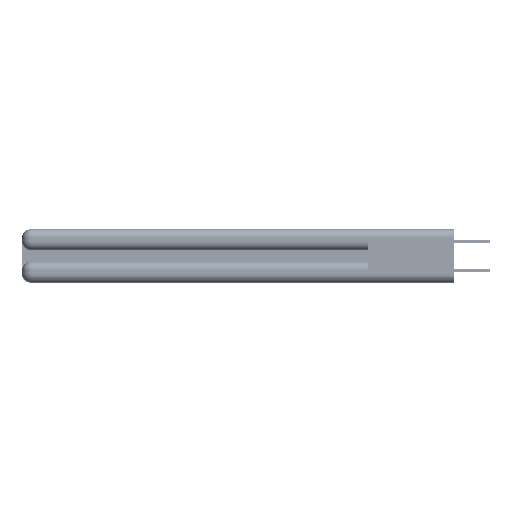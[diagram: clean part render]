
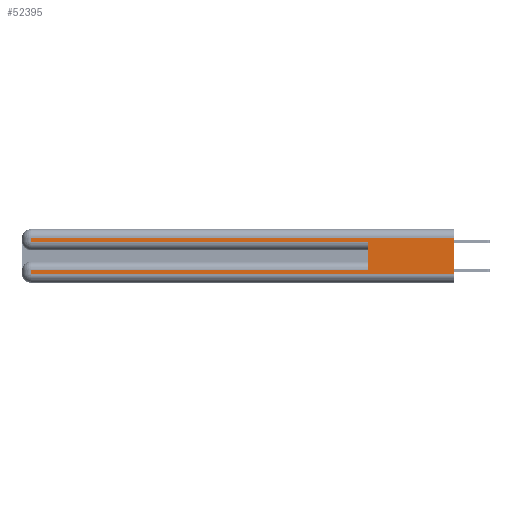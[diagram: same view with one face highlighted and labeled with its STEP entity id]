
A CAD part, left-side view. The second image highlights one B-rep face of the part: STEP entity #52395.
In plain terms, the highlighted planar face has unit normal (-1, 0, 0).
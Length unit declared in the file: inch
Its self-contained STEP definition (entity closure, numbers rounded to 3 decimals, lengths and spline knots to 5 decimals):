
#705 = CARTESIAN_POINT ( 'NONE',  ( 0., 0., 0.085 ) ) ;
#1115 = CARTESIAN_POINT ( 'NONE',  ( 0., 2.94, 0.37 ) ) ;
#1742 = DIRECTION ( 'NONE',  ( 0., 1., 0. ) ) ;
#2378 = VECTOR ( 'NONE', #22180, 39.37008 ) ;
#3705 = ORIENTED_EDGE ( 'NONE', *, *, #5007, .F. ) ;
#4146 = VERTEX_POINT ( 'NONE', #29857 ) ;
#4688 = DIRECTION ( 'NONE',  ( 1., 0., 0. ) ) ;
#5005 = VERTEX_POINT ( 'NONE', #43835 ) ;
#5007 = EDGE_CURVE ( 'NONE', #45916, #56265, #9834, .T. ) ;
#7320 = EDGE_CURVE ( 'NONE', #31704, #20163, #23789, .T. ) ;
#8880 = CARTESIAN_POINT ( 'NONE',  ( 0., 0.6, 0.145 ) ) ;
#9250 = PLANE ( 'NONE',  #31432 ) ;
#9301 = VECTOR ( 'NONE', #55175, 39.37008 ) ;
#9562 = CARTESIAN_POINT ( 'NONE',  ( 0., 2.94, 0.085 ) ) ;
#9834 = LINE ( 'NONE', #8880, #2378 ) ;
#10507 = ORIENTED_EDGE ( 'NONE', *, *, #16916, .T. ) ;
#10761 = CARTESIAN_POINT ( 'NONE',  ( 0., 0., 0.285 ) ) ;
#11599 = ORIENTED_EDGE ( 'NONE', *, *, #7320, .T. ) ;
#13138 = ORIENTED_EDGE ( 'NONE', *, *, #31001, .T. ) ;
#13433 = DIRECTION ( 'NONE',  ( 0., 0., -1. ) ) ;
#13495 = ORIENTED_EDGE ( 'NONE', *, *, #27789, .F. ) ;
#13810 = DIRECTION ( 'NONE',  ( 0., 1., 0. ) ) ;
#15706 = VECTOR ( 'NONE', #40473, 39.37008 ) ;
#16916 = EDGE_CURVE ( 'NONE', #33197, #56265, #39245, .T. ) ;
#17334 = CARTESIAN_POINT ( 'NONE',  ( 0., 0., 0.06 ) ) ;
#18394 = DIRECTION ( 'NONE',  ( 0., 0., -1. ) ) ;
#18413 = LINE ( 'NONE', #1115, #15706 ) ;
#18759 = CARTESIAN_POINT ( 'NONE',  ( 0., 0., 0.37 ) ) ;
#20163 = VERTEX_POINT ( 'NONE', #44011 ) ;
#22098 = LINE ( 'NONE', #27802, #38376 ) ;
#22180 = DIRECTION ( 'NONE',  ( 0., 0., 1. ) ) ;
#23002 = LINE ( 'NONE', #18759, #35207 ) ;
#23789 = LINE ( 'NONE', #43798, #40085 ) ;
#26553 = CARTESIAN_POINT ( 'NONE',  ( 0., 0., 0.37 ) ) ;
#27789 = EDGE_CURVE ( 'NONE', #55184, #4146, #23002, .T. ) ;
#27802 = CARTESIAN_POINT ( 'NONE',  ( 0., 0., 0.31 ) ) ;
#27840 = EDGE_LOOP ( 'NONE', ( #13495, #29357, #37471, #10507, #3705, #13138, #11599, #28764 ) ) ;
#28746 = EDGE_CURVE ( 'NONE', #20163, #4146, #48695, .T. ) ;
#28764 = ORIENTED_EDGE ( 'NONE', *, *, #28746, .T. ) ;
#29357 = ORIENTED_EDGE ( 'NONE', *, *, #53196, .T. ) ;
#29857 = CARTESIAN_POINT ( 'NONE',  ( 0., 0., 0.06 ) ) ;
#30088 = CARTESIAN_POINT ( 'NONE',  ( 0., 0., 0.31 ) ) ;
#30915 = FACE_OUTER_BOUND ( 'NONE', #27840, .T. ) ;
#31001 = EDGE_CURVE ( 'NONE', #45916, #31704, #46957, .T. ) ;
#31432 = AXIS2_PLACEMENT_3D ( 'NONE', #26553, #4688, #13433 ) ;
#31704 = VERTEX_POINT ( 'NONE', #9562 ) ;
#32636 = CARTESIAN_POINT ( 'NONE',  ( 0., 0.6, 0.285 ) ) ;
#33059 = VECTOR ( 'NONE', #38817, 39.37008 ) ;
#33197 = VERTEX_POINT ( 'NONE', #41361 ) ;
#35207 = VECTOR ( 'NONE', #18394, 39.37008 ) ;
#37471 = ORIENTED_EDGE ( 'NONE', *, *, #48840, .T. ) ;
#38376 = VECTOR ( 'NONE', #1742, 39.37008 ) ;
#38817 = DIRECTION ( 'NONE',  ( 0., -1., 0. ) ) ;
#39245 = LINE ( 'NONE', #10761, #9301 ) ;
#40085 = VECTOR ( 'NONE', #52514, 39.37008 ) ;
#40473 = DIRECTION ( 'NONE',  ( 0., 0., -1. ) ) ;
#41361 = CARTESIAN_POINT ( 'NONE',  ( 0., 2.94, 0.285 ) ) ;
#43798 = CARTESIAN_POINT ( 'NONE',  ( 0., 2.94, 0.37 ) ) ;
#43835 = CARTESIAN_POINT ( 'NONE',  ( 0., 2.94, 0.31 ) ) ;
#44011 = CARTESIAN_POINT ( 'NONE',  ( 0., 2.94, 0.06 ) ) ;
#45916 = VERTEX_POINT ( 'NONE', #46767 ) ;
#46767 = CARTESIAN_POINT ( 'NONE',  ( 0., 0.6, 0.085 ) ) ;
#46957 = LINE ( 'NONE', #705, #55783 ) ;
#48695 = LINE ( 'NONE', #17334, #33059 ) ;
#48840 = EDGE_CURVE ( 'NONE', #5005, #33197, #18413, .T. ) ;
#52395 = ADVANCED_FACE ( 'NONE', ( #30915 ), #9250, .F. ) ;
#52514 = DIRECTION ( 'NONE',  ( 0., 0., -1. ) ) ;
#53196 = EDGE_CURVE ( 'NONE', #55184, #5005, #22098, .T. ) ;
#55175 = DIRECTION ( 'NONE',  ( 0., -1., 0. ) ) ;
#55184 = VERTEX_POINT ( 'NONE', #30088 ) ;
#55783 = VECTOR ( 'NONE', #13810, 39.37008 ) ;
#56265 = VERTEX_POINT ( 'NONE', #32636 ) ;
